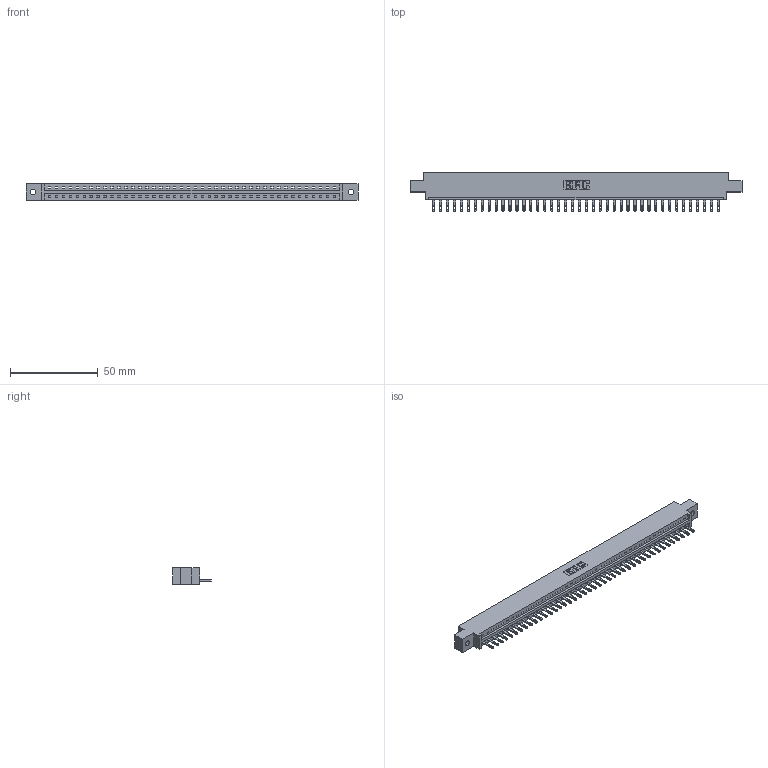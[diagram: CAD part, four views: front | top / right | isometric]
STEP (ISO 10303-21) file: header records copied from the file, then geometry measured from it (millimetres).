
FILE_DESCRIPTION (( 'STEP AP203' ), '1' );
FILE_NAME ('337-042-500-602.STEP', '2019-10-01T21:31:22', ( '' ), ( '' ), 'SwSTEP 2.0', 'SolidWorks 2016', '' );
FILE_SCHEMA (( 'CONFIG_CONTROL_DESIGN' ));
Length unit declared in the file: inch
Products named in the file (3): 345-292-001_345-293-100; 337-042-500-602; 337 Part_0.170 Offset - 0.128 Dia
Assembly tree (43 placements, depth 2):
  337-042-500-602
    337 Part_0.170 Offset - 0.128 Dia
    345-292-001_345-293-100  x42
Bounding box: 189.43 x 21.85 x 9.4 mm (x, y, z)
Volume: 19560.2 mm3; surface area: 20137.2 mm2
Topology: 43 solids, 43 shells, 2554 faces, 7883 edges, 5254 vertices
Faces by surface type: plane 1754, cylinder 800
Entity records: 31285 total; most frequent: CARTESIAN_POINT 5456, ORIENTED_EDGE 5434, DIRECTION 4593, EDGE_CURVE 2717, LINE 2585, VECTOR 2585, VERTEX_POINT 1810, AXIS2_PLACEMENT_3D 1004
